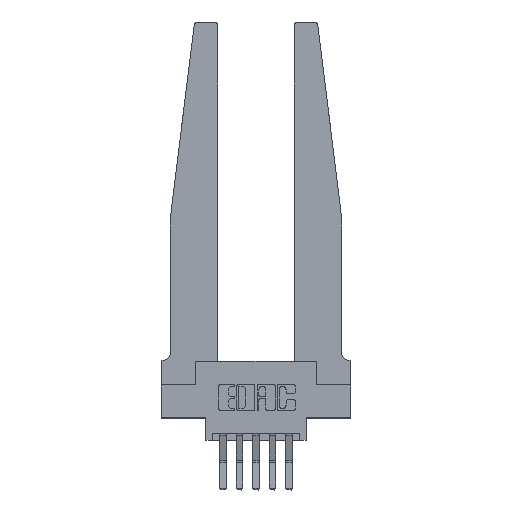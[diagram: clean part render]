
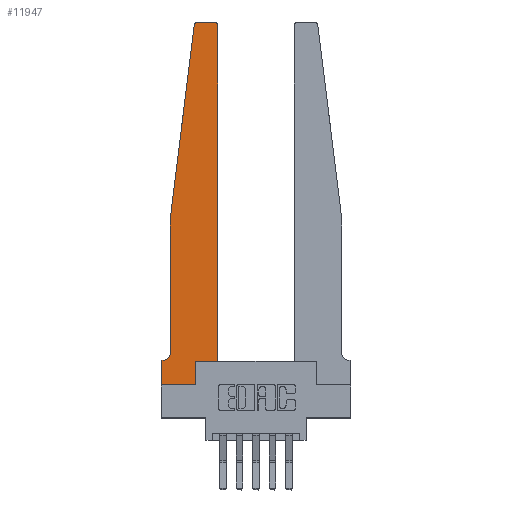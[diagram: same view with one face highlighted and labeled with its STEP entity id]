
A CAD part, top view. The second image highlights one B-rep face of the part: STEP entity #11947.
In plain terms, the highlighted planar face has unit normal (0, 0, 1).
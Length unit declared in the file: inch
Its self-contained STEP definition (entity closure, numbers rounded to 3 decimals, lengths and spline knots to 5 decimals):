
#46 = CARTESIAN_POINT ( 'NONE',  ( 0.2605, 0.18, 0.37 ) ) ;
#515 = DIRECTION ( 'NONE',  ( 1., 0., 0. ) ) ;
#607 = DIRECTION ( 'NONE',  ( 0., 0., -1. ) ) ;
#758 = VECTOR ( 'NONE', #4974, 39.37008 ) ;
#844 = CARTESIAN_POINT ( 'NONE',  ( 0., 0., 0.37 ) ) ;
#964 = CARTESIAN_POINT ( 'NONE',  ( 0.425, 0.18, 0.37 ) ) ;
#983 = ORIENTED_EDGE ( 'NONE', *, *, #12312, .T. ) ;
#1123 = LINE ( 'NONE', #5356, #5485 ) ;
#1128 = DIRECTION ( 'NONE',  ( -1., 0., 0. ) ) ;
#1196 = EDGE_CURVE ( 'NONE', #12555, #12732, #3134, .T. ) ;
#1214 = CIRCLE ( 'NONE', #6953, 0.05 ) ;
#1219 = ORIENTED_EDGE ( 'NONE', *, *, #7359, .T. ) ;
#1225 = CARTESIAN_POINT ( 'NONE',  ( 0.24675, 2.72367, 0.37 ) ) ;
#1369 = DIRECTION ( 'NONE',  ( 0., 0., 1. ) ) ;
#1471 = LINE ( 'NONE', #4533, #5966 ) ;
#1670 = LINE ( 'NONE', #844, #10589 ) ;
#1706 = LINE ( 'NONE', #2906, #758 ) ;
#1765 = EDGE_LOOP ( 'NONE', ( #11540, #13308, #11909, #5314, #11678, #1219, #5270, #1835, #983, #3133, #6792, #11413 ) ) ;
#1826 = CARTESIAN_POINT ( 'NONE',  ( 0.2605, 0., 0.37 ) ) ;
#1835 = ORIENTED_EDGE ( 'NONE', *, *, #7488, .T. ) ;
#1871 = CARTESIAN_POINT ( 'NONE',  ( 0.015, 0.1875, 0.37 ) ) ;
#1886 = DIRECTION ( 'NONE',  ( 0., 0., 1. ) ) ;
#1993 = CARTESIAN_POINT ( 'NONE',  ( 0.395, 2.72, 0.37 ) ) ;
#2038 = CARTESIAN_POINT ( 'NONE',  ( 0.065, 0.1875, 0.37 ) ) ;
#2075 = CARTESIAN_POINT ( 'NONE',  ( 0., 0.1875, 0.37 ) ) ;
#2109 = VERTEX_POINT ( 'NONE', #8409 ) ;
#2571 = AXIS2_PLACEMENT_3D ( 'NONE', #11297, #1886, #6121 ) ;
#2718 = CARTESIAN_POINT ( 'NONE',  ( 0.065, 1.25, 0.37 ) ) ;
#2878 = VERTEX_POINT ( 'NONE', #1871 ) ;
#2906 = CARTESIAN_POINT ( 'NONE',  ( 0.065, 1.25, 0.37 ) ) ;
#2999 = DIRECTION ( 'NONE',  ( 0., -1., 0. ) ) ;
#3092 = VERTEX_POINT ( 'NONE', #1225 ) ;
#3133 = ORIENTED_EDGE ( 'NONE', *, *, #8079, .T. ) ;
#3134 = LINE ( 'NONE', #9482, #3157 ) ;
#3157 = VECTOR ( 'NONE', #6239, 39.37008 ) ;
#3568 = VECTOR ( 'NONE', #1128, 39.37008 ) ;
#3684 = VERTEX_POINT ( 'NONE', #1826 ) ;
#3754 = VERTEX_POINT ( 'NONE', #5923 ) ;
#3836 = EDGE_CURVE ( 'NONE', #7173, #2109, #1123, .T. ) ;
#4264 = DIRECTION ( 'NONE',  ( 0., 1., 0. ) ) ;
#4533 = CARTESIAN_POINT ( 'NONE',  ( 0., 0., 0.37 ) ) ;
#4636 = DIRECTION ( 'NONE',  ( 1., 0., 0. ) ) ;
#4651 = CARTESIAN_POINT ( 'NONE',  ( 0.015, 0.2375, 0.37 ) ) ;
#4838 = DIRECTION ( 'NONE',  ( -1., 0., 0. ) ) ;
#4974 = DIRECTION ( 'NONE',  ( -0.122, -0.992, 0. ) ) ;
#4985 = VERTEX_POINT ( 'NONE', #2075 ) ;
#5131 = EDGE_CURVE ( 'NONE', #3754, #7643, #13424, .T. ) ;
#5270 = ORIENTED_EDGE ( 'NONE', *, *, #7593, .T. ) ;
#5314 = ORIENTED_EDGE ( 'NONE', *, *, #1196, .T. ) ;
#5356 = CARTESIAN_POINT ( 'NONE',  ( 0.25, 2.75, 0.37 ) ) ;
#5485 = VECTOR ( 'NONE', #6537, 39.37008 ) ;
#5606 = PLANE ( 'NONE',  #9385 ) ;
#5923 = CARTESIAN_POINT ( 'NONE',  ( 0.425, 0.18, 0.37 ) ) ;
#5966 = VECTOR ( 'NONE', #515, 39.37008 ) ;
#6010 = VERTEX_POINT ( 'NONE', #10675 ) ;
#6121 = DIRECTION ( 'NONE',  ( 1., 0., 0. ) ) ;
#6227 = CARTESIAN_POINT ( 'NONE',  ( 0.2605, 0.18, 0.37 ) ) ;
#6239 = DIRECTION ( 'NONE',  ( 0., -1., 0. ) ) ;
#6419 = VECTOR ( 'NONE', #12724, 39.37008 ) ;
#6537 = DIRECTION ( 'NONE',  ( -1., 0., 0. ) ) ;
#6752 = CIRCLE ( 'NONE', #2571, 0.03 ) ;
#6771 = CARTESIAN_POINT ( 'NONE',  ( 0.065, 0.2375, 0.37 ) ) ;
#6792 = ORIENTED_EDGE ( 'NONE', *, *, #5131, .T. ) ;
#6850 = VERTEX_POINT ( 'NONE', #6227 ) ;
#6953 = AXIS2_PLACEMENT_3D ( 'NONE', #4651, #607, #4838 ) ;
#7173 = VERTEX_POINT ( 'NONE', #11440 ) ;
#7359 = EDGE_CURVE ( 'NONE', #2878, #4985, #11510, .T. ) ;
#7488 = EDGE_CURVE ( 'NONE', #6010, #3684, #1471, .T. ) ;
#7593 = EDGE_CURVE ( 'NONE', #4985, #6010, #1670, .T. ) ;
#7603 = FACE_OUTER_BOUND ( 'NONE', #1765, .T. ) ;
#7643 = VERTEX_POINT ( 'NONE', #11140 ) ;
#7838 = AXIS2_PLACEMENT_3D ( 'NONE', #1993, #13476, #10639 ) ;
#8079 = EDGE_CURVE ( 'NONE', #6850, #3754, #8434, .T. ) ;
#8409 = CARTESIAN_POINT ( 'NONE',  ( 0.27653, 2.75, 0.37 ) ) ;
#8434 = LINE ( 'NONE', #964, #6419 ) ;
#9061 = EDGE_CURVE ( 'NONE', #3092, #12555, #1706, .T. ) ;
#9385 = AXIS2_PLACEMENT_3D ( 'NONE', #12015, #1369, #4636 ) ;
#9482 = CARTESIAN_POINT ( 'NONE',  ( 0.065, 1.25, 0.37 ) ) ;
#9984 = DIRECTION ( 'NONE',  ( 0., 1., 0. ) ) ;
#10260 = CIRCLE ( 'NONE', #7838, 0.03 ) ;
#10415 = LINE ( 'NONE', #46, #10717 ) ;
#10589 = VECTOR ( 'NONE', #2999, 39.37008 ) ;
#10639 = DIRECTION ( 'NONE',  ( 1., 0., 0. ) ) ;
#10675 = CARTESIAN_POINT ( 'NONE',  ( 0., 0., 0.37 ) ) ;
#10717 = VECTOR ( 'NONE', #4264, 39.37008 ) ;
#11140 = CARTESIAN_POINT ( 'NONE',  ( 0.425, 2.72, 0.37 ) ) ;
#11193 = EDGE_CURVE ( 'NONE', #2109, #3092, #6752, .T. ) ;
#11297 = CARTESIAN_POINT ( 'NONE',  ( 0.27653, 2.72, 0.37 ) ) ;
#11413 = ORIENTED_EDGE ( 'NONE', *, *, #11775, .T. ) ;
#11440 = CARTESIAN_POINT ( 'NONE',  ( 0.395, 2.75, 0.37 ) ) ;
#11510 = LINE ( 'NONE', #2038, #3568 ) ;
#11540 = ORIENTED_EDGE ( 'NONE', *, *, #3836, .T. ) ;
#11668 = VECTOR ( 'NONE', #9984, 39.37008 ) ;
#11678 = ORIENTED_EDGE ( 'NONE', *, *, #12637, .T. ) ;
#11775 = EDGE_CURVE ( 'NONE', #7643, #7173, #10260, .T. ) ;
#11909 = ORIENTED_EDGE ( 'NONE', *, *, #9061, .T. ) ;
#11947 = ADVANCED_FACE ( 'NONE', ( #7603 ), #5606, .T. ) ;
#12015 = CARTESIAN_POINT ( 'NONE',  ( 0., 0.1875, 0.37 ) ) ;
#12312 = EDGE_CURVE ( 'NONE', #3684, #6850, #10415, .T. ) ;
#12555 = VERTEX_POINT ( 'NONE', #2718 ) ;
#12637 = EDGE_CURVE ( 'NONE', #12732, #2878, #1214, .T. ) ;
#12724 = DIRECTION ( 'NONE',  ( 1., 0., 0. ) ) ;
#12732 = VERTEX_POINT ( 'NONE', #6771 ) ;
#13285 = CARTESIAN_POINT ( 'NONE',  ( 0.425, 0.18, 0.37 ) ) ;
#13308 = ORIENTED_EDGE ( 'NONE', *, *, #11193, .T. ) ;
#13424 = LINE ( 'NONE', #13285, #11668 ) ;
#13476 = DIRECTION ( 'NONE',  ( 0., 0., 1. ) ) ;
